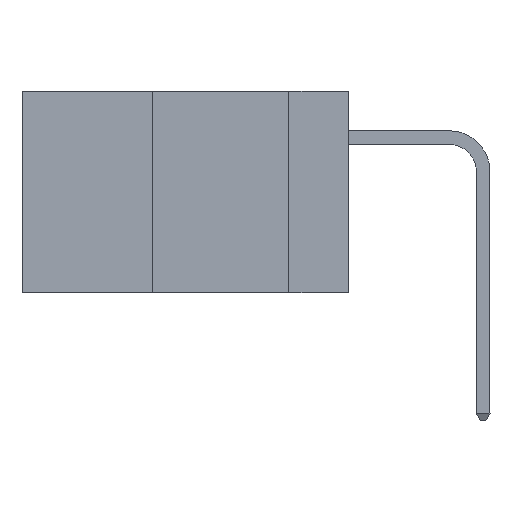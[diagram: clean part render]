
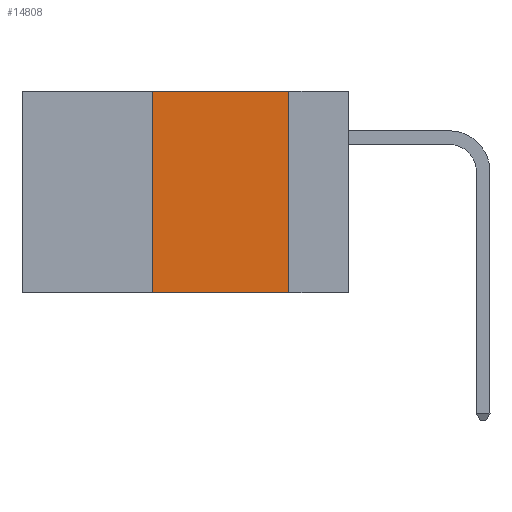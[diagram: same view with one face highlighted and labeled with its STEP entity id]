
A CAD part, left-side view. The second image highlights one B-rep face of the part: STEP entity #14808.
In plain terms, the highlighted planar face has unit normal (-1, 0, 0).
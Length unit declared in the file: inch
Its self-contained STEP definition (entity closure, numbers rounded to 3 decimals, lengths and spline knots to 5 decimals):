
#448 = VECTOR ( 'NONE', #2811, 39.37008 ) ;
#763 = VERTEX_POINT ( 'NONE', #872 ) ;
#872 = CARTESIAN_POINT ( 'NONE',  ( 0., 0.11, -0.37 ) ) ;
#950 = EDGE_CURVE ( 'NONE', #2138, #763, #3724, .T. ) ;
#1019 = LINE ( 'NONE', #13649, #13940 ) ;
#1340 = EDGE_CURVE ( 'NONE', #14407, #8229, #2643, .T. ) ;
#2138 = VERTEX_POINT ( 'NONE', #2361 ) ;
#2302 = CARTESIAN_POINT ( 'NONE',  ( 0., 0.11, 0. ) ) ;
#2361 = CARTESIAN_POINT ( 'NONE',  ( 0., 0.11, 0. ) ) ;
#2643 = LINE ( 'NONE', #10509, #11297 ) ;
#2811 = DIRECTION ( 'NONE',  ( 0., 0., -1. ) ) ;
#2907 = EDGE_LOOP ( 'NONE', ( #7584, #8049, #13742, #6668 ) ) ;
#3296 = DIRECTION ( 'NONE',  ( 0., -1., 0. ) ) ;
#3586 = DIRECTION ( 'NONE',  ( 0., 0., -1. ) ) ;
#3724 = LINE ( 'NONE', #2302, #448 ) ;
#3738 = DIRECTION ( 'NONE',  ( 1., 0., 0. ) ) ;
#4669 = AXIS2_PLACEMENT_3D ( 'NONE', #4878, #3738, #3586 ) ;
#4878 = CARTESIAN_POINT ( 'NONE',  ( 0., 0.6, 0. ) ) ;
#5680 = EDGE_CURVE ( 'NONE', #14407, #763, #1019, .T. ) ;
#6058 = CARTESIAN_POINT ( 'NONE',  ( 0., 0.36, -0.37 ) ) ;
#6668 = ORIENTED_EDGE ( 'NONE', *, *, #5680, .T. ) ;
#7273 = DIRECTION ( 'NONE',  ( 0., 0., 1. ) ) ;
#7584 = ORIENTED_EDGE ( 'NONE', *, *, #950, .F. ) ;
#8049 = ORIENTED_EDGE ( 'NONE', *, *, #10827, .F. ) ;
#8229 = VERTEX_POINT ( 'NONE', #10873 ) ;
#8284 = PLANE ( 'NONE',  #4669 ) ;
#8442 = FACE_OUTER_BOUND ( 'NONE', #2907, .T. ) ;
#8469 = LINE ( 'NONE', #12970, #12136 ) ;
#10509 = CARTESIAN_POINT ( 'NONE',  ( 0., 0.36, 0. ) ) ;
#10715 = DIRECTION ( 'NONE',  ( 0., -1., 0. ) ) ;
#10827 = EDGE_CURVE ( 'NONE', #8229, #2138, #8469, .T. ) ;
#10873 = CARTESIAN_POINT ( 'NONE',  ( 0., 0.36, 0. ) ) ;
#11297 = VECTOR ( 'NONE', #7273, 39.37008 ) ;
#12136 = VECTOR ( 'NONE', #10715, 39.37008 ) ;
#12970 = CARTESIAN_POINT ( 'NONE',  ( 0., 0.6, 0. ) ) ;
#13649 = CARTESIAN_POINT ( 'NONE',  ( 0., 0.6, -0.37 ) ) ;
#13742 = ORIENTED_EDGE ( 'NONE', *, *, #1340, .F. ) ;
#13940 = VECTOR ( 'NONE', #3296, 39.37008 ) ;
#14407 = VERTEX_POINT ( 'NONE', #6058 ) ;
#14808 = ADVANCED_FACE ( 'NONE', ( #8442 ), #8284, .F. ) ;
